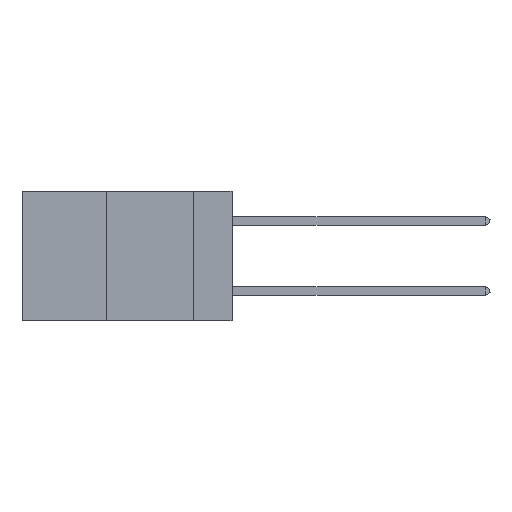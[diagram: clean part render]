
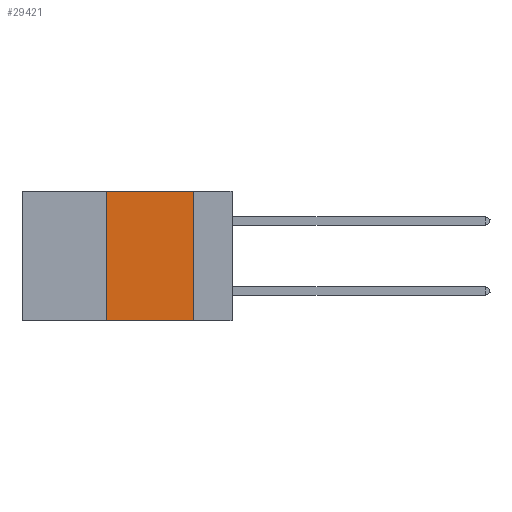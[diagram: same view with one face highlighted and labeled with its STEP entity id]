
A CAD part, left-side view. The second image highlights one B-rep face of the part: STEP entity #29421.
In plain terms, the highlighted planar face has unit normal (-1, 0, 0).
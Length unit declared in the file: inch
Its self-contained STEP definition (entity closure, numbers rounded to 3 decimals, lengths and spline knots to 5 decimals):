
#1702 = AXIS2_PLACEMENT_3D ( 'NONE', #21968, #7559, #24315 ) ;
#3447 = ORIENTED_EDGE ( 'NONE', *, *, #21595, .T. ) ;
#4399 = LINE ( 'NONE', #6351, #22876 ) ;
#5527 = VERTEX_POINT ( 'NONE', #12352 ) ;
#6351 = CARTESIAN_POINT ( 'NONE',  ( 0., 0.6, -0.37 ) ) ;
#7559 = DIRECTION ( 'NONE',  ( 1., 0., 0. ) ) ;
#8187 = CARTESIAN_POINT ( 'NONE',  ( 0., 0.6, 0. ) ) ;
#9283 = FACE_OUTER_BOUND ( 'NONE', #17438, .T. ) ;
#10399 = VECTOR ( 'NONE', #20190, 39.37008 ) ;
#10551 = VERTEX_POINT ( 'NONE', #15927 ) ;
#12352 = CARTESIAN_POINT ( 'NONE',  ( 0., 0.11, -0.37 ) ) ;
#12489 = DIRECTION ( 'NONE',  ( 0., 0., -1. ) ) ;
#13106 = CARTESIAN_POINT ( 'NONE',  ( 0., 0.36, 0. ) ) ;
#14934 = CARTESIAN_POINT ( 'NONE',  ( 0., 0.11, 0. ) ) ;
#15546 = DIRECTION ( 'NONE',  ( 0., 0., 1. ) ) ;
#15927 = CARTESIAN_POINT ( 'NONE',  ( 0., 0.11, 0. ) ) ;
#15947 = DIRECTION ( 'NONE',  ( 0., -1., 0. ) ) ;
#16818 = VECTOR ( 'NONE', #12489, 39.37008 ) ;
#17162 = PLANE ( 'NONE',  #1702 ) ;
#17438 = EDGE_LOOP ( 'NONE', ( #22032, #20155, #30747, #3447 ) ) ;
#17561 = VERTEX_POINT ( 'NONE', #27476 ) ;
#17566 = LINE ( 'NONE', #14934, #16818 ) ;
#17684 = LINE ( 'NONE', #13106, #29551 ) ;
#20155 = ORIENTED_EDGE ( 'NONE', *, *, #29581, .F. ) ;
#20190 = DIRECTION ( 'NONE',  ( 0., -1., 0. ) ) ;
#21595 = EDGE_CURVE ( 'NONE', #26613, #5527, #4399, .T. ) ;
#21968 = CARTESIAN_POINT ( 'NONE',  ( 0., 0.6, 0. ) ) ;
#22032 = ORIENTED_EDGE ( 'NONE', *, *, #22679, .F. ) ;
#22402 = CARTESIAN_POINT ( 'NONE',  ( 0., 0.36, -0.37 ) ) ;
#22679 = EDGE_CURVE ( 'NONE', #10551, #5527, #17566, .T. ) ;
#22876 = VECTOR ( 'NONE', #15947, 39.37008 ) ;
#23883 = LINE ( 'NONE', #8187, #10399 ) ;
#24315 = DIRECTION ( 'NONE',  ( 0., 0., -1. ) ) ;
#26613 = VERTEX_POINT ( 'NONE', #22402 ) ;
#27476 = CARTESIAN_POINT ( 'NONE',  ( 0., 0.36, 0. ) ) ;
#27777 = EDGE_CURVE ( 'NONE', #26613, #17561, #17684, .T. ) ;
#29421 = ADVANCED_FACE ( 'NONE', ( #9283 ), #17162, .F. ) ;
#29551 = VECTOR ( 'NONE', #15546, 39.37008 ) ;
#29581 = EDGE_CURVE ( 'NONE', #17561, #10551, #23883, .T. ) ;
#30747 = ORIENTED_EDGE ( 'NONE', *, *, #27777, .F. ) ;
